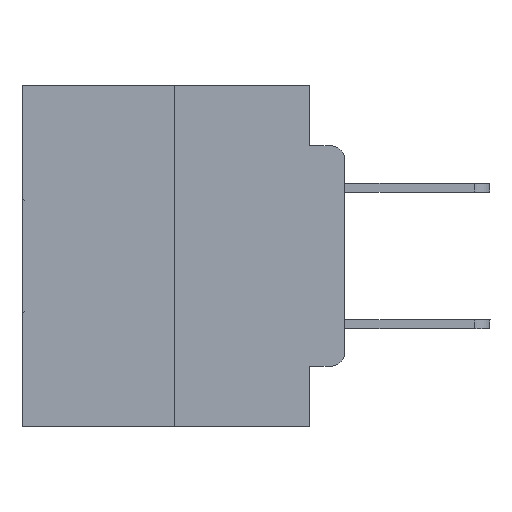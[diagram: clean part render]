
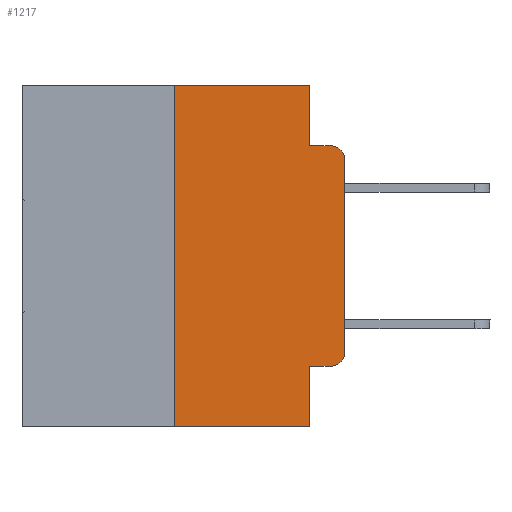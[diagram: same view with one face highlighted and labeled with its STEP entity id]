
A CAD part, left-side view. The second image highlights one B-rep face of the part: STEP entity #1217.
In plain terms, the highlighted planar face has unit normal (-1, 0, 0).
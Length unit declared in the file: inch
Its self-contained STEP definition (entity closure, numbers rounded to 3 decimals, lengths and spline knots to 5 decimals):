
#144 = CARTESIAN_POINT ( 'NONE',  ( 0., 0.02, -0.1085 ) ) ;
#205 = CARTESIAN_POINT ( 'NONE',  ( 0., 0.051, 0. ) ) ;
#352 = ORIENTED_EDGE ( 'NONE', *, *, #2902, .F. ) ;
#589 = VERTEX_POINT ( 'NONE', #25706 ) ;
#850 = DIRECTION ( 'NONE',  ( 0., 0., -1. ) ) ;
#919 = ORIENTED_EDGE ( 'NONE', *, *, #5625, .F. ) ;
#977 = VECTOR ( 'NONE', #30178, 39.37008 ) ;
#1217 = ADVANCED_FACE ( 'NONE', ( #7519 ), #19243, .F. ) ;
#2192 = DIRECTION ( 'NONE',  ( 0., 0., -1. ) ) ;
#2411 = CIRCLE ( 'NONE', #11409, 0.02 ) ;
#2616 = EDGE_CURVE ( 'NONE', #9592, #6085, #16609, .T. ) ;
#2902 = EDGE_CURVE ( 'NONE', #20474, #26999, #6726, .T. ) ;
#3890 = LINE ( 'NONE', #18417, #24750 ) ;
#3919 = CARTESIAN_POINT ( 'NONE',  ( 0., 0.25, 0. ) ) ;
#4019 = CARTESIAN_POINT ( 'NONE',  ( 0., 0.02, -0.4115 ) ) ;
#4940 = CARTESIAN_POINT ( 'NONE',  ( 0., 0.25, -0.5 ) ) ;
#5284 = LINE ( 'NONE', #29162, #5377 ) ;
#5377 = VECTOR ( 'NONE', #11995, 39.37008 ) ;
#5625 = EDGE_CURVE ( 'NONE', #8289, #17910, #5284, .T. ) ;
#6040 = ORIENTED_EDGE ( 'NONE', *, *, #28835, .T. ) ;
#6085 = VERTEX_POINT ( 'NONE', #18840 ) ;
#6303 = EDGE_CURVE ( 'NONE', #589, #8289, #22095, .T. ) ;
#6336 = VERTEX_POINT ( 'NONE', #25704 ) ;
#6726 = LINE ( 'NONE', #3919, #24265 ) ;
#6788 = AXIS2_PLACEMENT_3D ( 'NONE', #12502, #18922, #14240 ) ;
#7103 = DIRECTION ( 'NONE',  ( 0., 0., -1. ) ) ;
#7304 = VERTEX_POINT ( 'NONE', #4019 ) ;
#7519 = FACE_OUTER_BOUND ( 'NONE', #23555, .T. ) ;
#7773 = DIRECTION ( 'NONE',  ( 0., -1., 0. ) ) ;
#8289 = VERTEX_POINT ( 'NONE', #26288 ) ;
#8392 = VECTOR ( 'NONE', #17074, 39.37008 ) ;
#9592 = VERTEX_POINT ( 'NONE', #18676 ) ;
#10083 = CARTESIAN_POINT ( 'NONE',  ( 0., 0.051, 0. ) ) ;
#10124 = ORIENTED_EDGE ( 'NONE', *, *, #30069, .F. ) ;
#10702 = EDGE_CURVE ( 'NONE', #9592, #7304, #28695, .T. ) ;
#11209 = VECTOR ( 'NONE', #850, 39.37008 ) ;
#11409 = AXIS2_PLACEMENT_3D ( 'NONE', #19008, #21352, #26157 ) ;
#11512 = EDGE_CURVE ( 'NONE', #20474, #6085, #26142, .T. ) ;
#11995 = DIRECTION ( 'NONE',  ( 0., -1., 0. ) ) ;
#12502 = CARTESIAN_POINT ( 'NONE',  ( 0., 0.473, 0. ) ) ;
#14240 = DIRECTION ( 'NONE',  ( 0., 0., -1. ) ) ;
#15488 = VERTEX_POINT ( 'NONE', #28937 ) ;
#15921 = DIRECTION ( 'NONE',  ( 0., 0., 1. ) ) ;
#16259 = CIRCLE ( 'NONE', #21735, 0.02 ) ;
#16413 = LINE ( 'NONE', #27836, #977 ) ;
#16548 = DIRECTION ( 'NONE',  ( -1., 0., 0. ) ) ;
#16609 = LINE ( 'NONE', #205, #22035 ) ;
#16842 = ORIENTED_EDGE ( 'NONE', *, *, #6303, .F. ) ;
#17074 = DIRECTION ( 'NONE',  ( 0., -1., 0. ) ) ;
#17264 = ORIENTED_EDGE ( 'NONE', *, *, #24203, .T. ) ;
#17910 = VERTEX_POINT ( 'NONE', #23789 ) ;
#18353 = ORIENTED_EDGE ( 'NONE', *, *, #2616, .F. ) ;
#18417 = CARTESIAN_POINT ( 'NONE',  ( 0., 0., 0. ) ) ;
#18676 = CARTESIAN_POINT ( 'NONE',  ( 0., 0.051, -0.4115 ) ) ;
#18840 = CARTESIAN_POINT ( 'NONE',  ( 0., 0.051, -0.5 ) ) ;
#18922 = DIRECTION ( 'NONE',  ( 1., 0., 0. ) ) ;
#19008 = CARTESIAN_POINT ( 'NONE',  ( 0., 0.02, -0.3915 ) ) ;
#19243 = PLANE ( 'NONE',  #6788 ) ;
#20474 = VERTEX_POINT ( 'NONE', #4940 ) ;
#20653 = ORIENTED_EDGE ( 'NONE', *, *, #10702, .T. ) ;
#21352 = DIRECTION ( 'NONE',  ( -1., 0., 0. ) ) ;
#21666 = CARTESIAN_POINT ( 'NONE',  ( 0., 0.051, -0.4115 ) ) ;
#21735 = AXIS2_PLACEMENT_3D ( 'NONE', #144, #16548, #2192 ) ;
#22035 = VECTOR ( 'NONE', #7103, 39.37008 ) ;
#22095 = LINE ( 'NONE', #10083, #11209 ) ;
#23274 = DIRECTION ( 'NONE',  ( 0., 0., 1. ) ) ;
#23555 = EDGE_LOOP ( 'NONE', ( #23603, #17264, #919, #16842, #10124, #352, #29331, #18353, #20653, #6040 ) ) ;
#23603 = ORIENTED_EDGE ( 'NONE', *, *, #24435, .T. ) ;
#23789 = CARTESIAN_POINT ( 'NONE',  ( 0., 0.02, -0.0885 ) ) ;
#24203 = EDGE_CURVE ( 'NONE', #15488, #17910, #16259, .T. ) ;
#24265 = VECTOR ( 'NONE', #23274, 39.37008 ) ;
#24435 = EDGE_CURVE ( 'NONE', #6336, #15488, #3890, .T. ) ;
#24750 = VECTOR ( 'NONE', #15921, 39.37008 ) ;
#25704 = CARTESIAN_POINT ( 'NONE',  ( 0., 0., -0.3915 ) ) ;
#25706 = CARTESIAN_POINT ( 'NONE',  ( 0., 0.051, 0. ) ) ;
#26142 = LINE ( 'NONE', #28626, #8392 ) ;
#26157 = DIRECTION ( 'NONE',  ( 0., 0., -1. ) ) ;
#26288 = CARTESIAN_POINT ( 'NONE',  ( 0., 0.051, -0.0885 ) ) ;
#26380 = CARTESIAN_POINT ( 'NONE',  ( 0., 0.25, 0. ) ) ;
#26999 = VERTEX_POINT ( 'NONE', #26380 ) ;
#27836 = CARTESIAN_POINT ( 'NONE',  ( 0., 0.473, 0. ) ) ;
#28626 = CARTESIAN_POINT ( 'NONE',  ( 0., 0.473, -0.5 ) ) ;
#28695 = LINE ( 'NONE', #21666, #29769 ) ;
#28835 = EDGE_CURVE ( 'NONE', #7304, #6336, #2411, .T. ) ;
#28937 = CARTESIAN_POINT ( 'NONE',  ( 0., 0., -0.1085 ) ) ;
#29162 = CARTESIAN_POINT ( 'NONE',  ( 0., 0.051, -0.0885 ) ) ;
#29331 = ORIENTED_EDGE ( 'NONE', *, *, #11512, .T. ) ;
#29769 = VECTOR ( 'NONE', #7773, 39.37008 ) ;
#30069 = EDGE_CURVE ( 'NONE', #26999, #589, #16413, .T. ) ;
#30178 = DIRECTION ( 'NONE',  ( 0., -1., 0. ) ) ;
